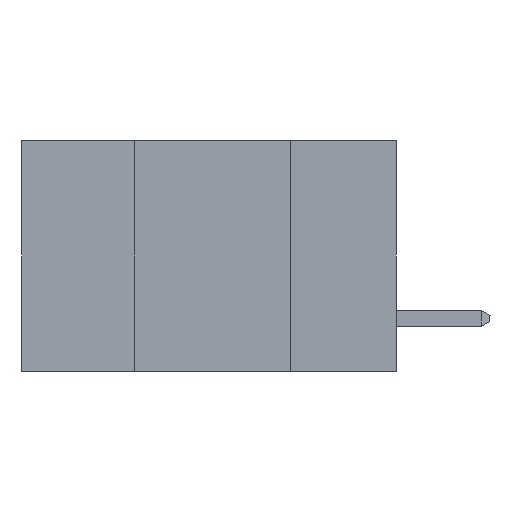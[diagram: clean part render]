
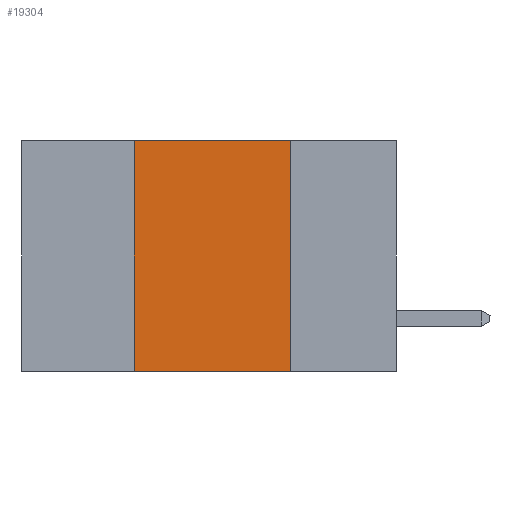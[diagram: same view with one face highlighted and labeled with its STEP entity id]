
A CAD part, left-side view. The second image highlights one B-rep face of the part: STEP entity #19304.
In plain terms, the highlighted planar face has unit normal (-1, 0, 0).
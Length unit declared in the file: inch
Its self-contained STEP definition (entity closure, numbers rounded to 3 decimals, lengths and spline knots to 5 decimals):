
#105 = DIRECTION ( 'NONE',  ( 0., -1., 0. ) ) ;
#322 = CARTESIAN_POINT ( 'NONE',  ( 0., 0.42, -0.37 ) ) ;
#623 = VECTOR ( 'NONE', #8601, 39.37008 ) ;
#706 = AXIS2_PLACEMENT_3D ( 'NONE', #16041, #11633, #2306 ) ;
#2306 = DIRECTION ( 'NONE',  ( 0., 0., -1. ) ) ;
#3781 = VERTEX_POINT ( 'NONE', #12692 ) ;
#4539 = LINE ( 'NONE', #18334, #16196 ) ;
#4836 = LINE ( 'NONE', #11644, #623 ) ;
#5241 = ORIENTED_EDGE ( 'NONE', *, *, #15169, .T. ) ;
#5663 = VECTOR ( 'NONE', #5732, 39.37008 ) ;
#5732 = DIRECTION ( 'NONE',  ( 0., -1., 0. ) ) ;
#5795 = VERTEX_POINT ( 'NONE', #11156 ) ;
#5934 = ORIENTED_EDGE ( 'NONE', *, *, #18102, .F. ) ;
#6958 = ORIENTED_EDGE ( 'NONE', *, *, #16190, .F. ) ;
#7004 = PLANE ( 'NONE',  #706 ) ;
#7192 = LINE ( 'NONE', #14718, #10814 ) ;
#8391 = FACE_OUTER_BOUND ( 'NONE', #17797, .T. ) ;
#8601 = DIRECTION ( 'NONE',  ( 0., 0., 1. ) ) ;
#9938 = VERTEX_POINT ( 'NONE', #12630 ) ;
#10299 = LINE ( 'NONE', #13384, #5663 ) ;
#10814 = VECTOR ( 'NONE', #16219, 39.37008 ) ;
#11156 = CARTESIAN_POINT ( 'NONE',  ( 0., 0.17, 0. ) ) ;
#11633 = DIRECTION ( 'NONE',  ( 1., 0., 0. ) ) ;
#11644 = CARTESIAN_POINT ( 'NONE',  ( 0., 0.42, -0.37 ) ) ;
#12630 = CARTESIAN_POINT ( 'NONE',  ( 0., 0.42, 0. ) ) ;
#12692 = CARTESIAN_POINT ( 'NONE',  ( 0., 0.17, -0.37 ) ) ;
#13384 = CARTESIAN_POINT ( 'NONE',  ( 0., 0.6, -0.37 ) ) ;
#14718 = CARTESIAN_POINT ( 'NONE',  ( 0., 0.17, -0.37 ) ) ;
#15169 = EDGE_CURVE ( 'NONE', #16695, #3781, #10299, .T. ) ;
#16041 = CARTESIAN_POINT ( 'NONE',  ( 0., 0.6, 0. ) ) ;
#16190 = EDGE_CURVE ( 'NONE', #16695, #9938, #4836, .T. ) ;
#16196 = VECTOR ( 'NONE', #105, 39.37008 ) ;
#16219 = DIRECTION ( 'NONE',  ( 0., 0., -1. ) ) ;
#16695 = VERTEX_POINT ( 'NONE', #322 ) ;
#17164 = EDGE_CURVE ( 'NONE', #9938, #5795, #4539, .T. ) ;
#17797 = EDGE_LOOP ( 'NONE', ( #5934, #18401, #6958, #5241 ) ) ;
#18102 = EDGE_CURVE ( 'NONE', #5795, #3781, #7192, .T. ) ;
#18334 = CARTESIAN_POINT ( 'NONE',  ( 0., 0.6, 0. ) ) ;
#18401 = ORIENTED_EDGE ( 'NONE', *, *, #17164, .F. ) ;
#19304 = ADVANCED_FACE ( 'NONE', ( #8391 ), #7004, .F. ) ;
